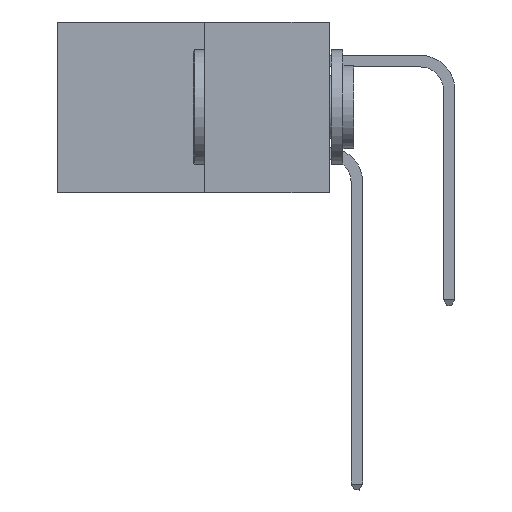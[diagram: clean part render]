
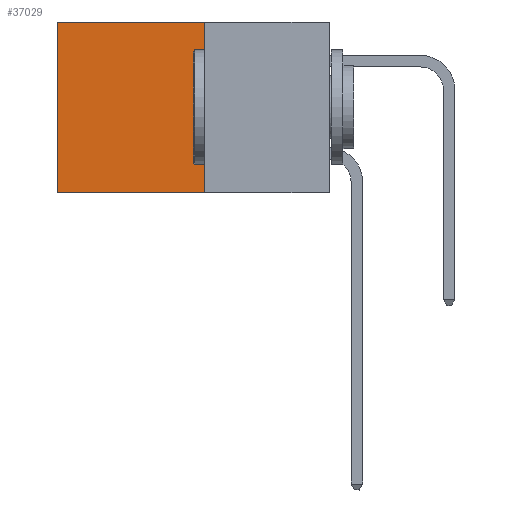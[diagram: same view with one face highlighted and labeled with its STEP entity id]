
A CAD part, left-side view. The second image highlights one B-rep face of the part: STEP entity #37029.
In plain terms, the highlighted planar face has unit normal (-1, 0, 0).
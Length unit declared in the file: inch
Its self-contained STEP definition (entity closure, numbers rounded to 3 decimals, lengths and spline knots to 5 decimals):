
#684 = DIRECTION ( 'NONE',  ( 0., 1., 0. ) ) ;
#1009 = CARTESIAN_POINT ( 'NONE',  ( 0.277, 0.27, -0.37 ) ) ;
#1249 = CARTESIAN_POINT ( 'NONE',  ( 0.277, 0.59, 0. ) ) ;
#3316 = FACE_OUTER_BOUND ( 'NONE', #30827, .T. ) ;
#3752 = CARTESIAN_POINT ( 'NONE',  ( 0.277, 0.59, -0.37 ) ) ;
#5269 = VECTOR ( 'NONE', #15956, 39.37008 ) ;
#6393 = VECTOR ( 'NONE', #6708, 39.37008 ) ;
#6708 = DIRECTION ( 'NONE',  ( 0., 0., -1. ) ) ;
#8566 = CARTESIAN_POINT ( 'NONE',  ( 0.277, 0.27, 0. ) ) ;
#10902 = CARTESIAN_POINT ( 'NONE',  ( 0.277, 0.27, -0.37 ) ) ;
#11748 = VERTEX_POINT ( 'NONE', #1249 ) ;
#11901 = CARTESIAN_POINT ( 'NONE',  ( 0.277, 0.27, -0.37 ) ) ;
#12697 = LINE ( 'NONE', #15297, #34811 ) ;
#12777 = LINE ( 'NONE', #10902, #20473 ) ;
#12956 = DIRECTION ( 'NONE',  ( 1., 0., 0. ) ) ;
#14600 = EDGE_CURVE ( 'NONE', #11748, #28899, #37103, .T. ) ;
#14645 = ORIENTED_EDGE ( 'NONE', *, *, #15327, .F. ) ;
#15297 = CARTESIAN_POINT ( 'NONE',  ( 0.277, 0.27, -0.37 ) ) ;
#15303 = AXIS2_PLACEMENT_3D ( 'NONE', #1009, #12956, #33152 ) ;
#15327 = EDGE_CURVE ( 'NONE', #17547, #28899, #12697, .T. ) ;
#15956 = DIRECTION ( 'NONE',  ( 0., 1., 0. ) ) ;
#17547 = VERTEX_POINT ( 'NONE', #11901 ) ;
#18923 = CARTESIAN_POINT ( 'NONE',  ( 0.277, 0.59, -0.37 ) ) ;
#20198 = EDGE_CURVE ( 'NONE', #24866, #11748, #28413, .T. ) ;
#20473 = VECTOR ( 'NONE', #28234, 39.37008 ) ;
#24866 = VERTEX_POINT ( 'NONE', #8566 ) ;
#28234 = DIRECTION ( 'NONE',  ( 0., 0., -1. ) ) ;
#28413 = LINE ( 'NONE', #30367, #5269 ) ;
#28899 = VERTEX_POINT ( 'NONE', #18923 ) ;
#29144 = ORIENTED_EDGE ( 'NONE', *, *, #20198, .T. ) ;
#30277 = PLANE ( 'NONE',  #15303 ) ;
#30367 = CARTESIAN_POINT ( 'NONE',  ( 0.277, 0.27, 0. ) ) ;
#30827 = EDGE_LOOP ( 'NONE', ( #35775, #14645, #32985, #29144 ) ) ;
#32985 = ORIENTED_EDGE ( 'NONE', *, *, #34576, .F. ) ;
#33152 = DIRECTION ( 'NONE',  ( 0., 0., -1. ) ) ;
#34576 = EDGE_CURVE ( 'NONE', #24866, #17547, #12777, .T. ) ;
#34811 = VECTOR ( 'NONE', #684, 39.37008 ) ;
#35775 = ORIENTED_EDGE ( 'NONE', *, *, #14600, .T. ) ;
#37029 = ADVANCED_FACE ( 'NONE', ( #3316 ), #30277, .F. ) ;
#37103 = LINE ( 'NONE', #3752, #6393 ) ;
